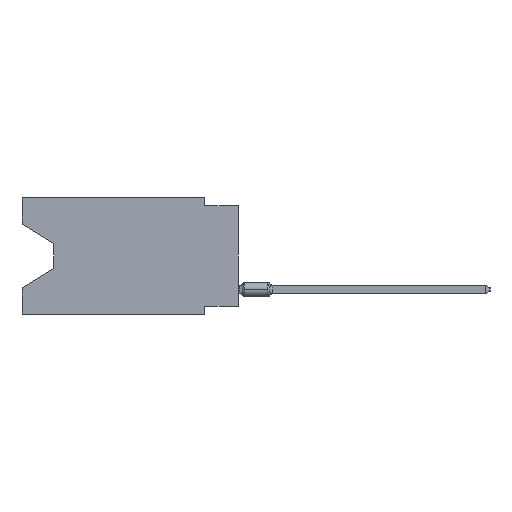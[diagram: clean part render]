
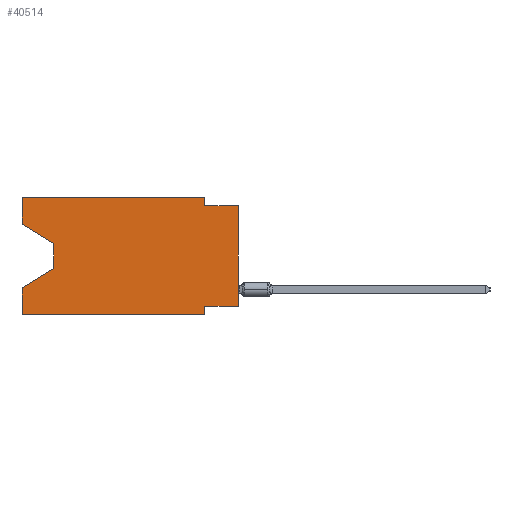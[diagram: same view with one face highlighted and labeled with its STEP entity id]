
A CAD part, left-side view. The second image highlights one B-rep face of the part: STEP entity #40514.
In plain terms, the highlighted planar face has unit normal (-1, 0, 0).
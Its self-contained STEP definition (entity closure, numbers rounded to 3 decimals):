
#3 = LINE ( 'NONE', #67822, #55058 ) ;
#1904 = DIRECTION ( 'NONE',  ( 0., -1., 0. ) ) ;
#2317 = ORIENTED_EDGE ( 'NONE', *, *, #14284, .F. ) ;
#2557 = VECTOR ( 'NONE', #18844, 1000. ) ;
#3692 = DIRECTION ( 'NONE',  ( 0., 0., -1. ) ) ;
#3915 = CARTESIAN_POINT ( 'NONE',  ( 0., 2.54, -8.255 ) ) ;
#7054 = CARTESIAN_POINT ( 'NONE',  ( 0., 0., -8.255 ) ) ;
#8529 = ORIENTED_EDGE ( 'NONE', *, *, #83714, .T. ) ;
#8626 = VECTOR ( 'NONE', #66168, 1000. ) ;
#8939 = DIRECTION ( 'NONE',  ( 0., 1., 0. ) ) ;
#9655 = VERTEX_POINT ( 'NONE', #47200 ) ;
#10917 = CARTESIAN_POINT ( 'NONE',  ( 0., 16.383, -2.038 ) ) ;
#12584 = CARTESIAN_POINT ( 'NONE',  ( 0., 16.383, 0. ) ) ;
#12741 = CARTESIAN_POINT ( 'NONE',  ( 0., 0., 0. ) ) ;
#12987 = ORIENTED_EDGE ( 'NONE', *, *, #36644, .F. ) ;
#13260 = LINE ( 'NONE', #43093, #8626 ) ;
#14284 = EDGE_CURVE ( 'NONE', #58173, #48306, #53150, .T. ) ;
#14728 = VERTEX_POINT ( 'NONE', #73076 ) ;
#16067 = VERTEX_POINT ( 'NONE', #92377 ) ;
#16090 = DIRECTION ( 'NONE',  ( 0., 0., 1. ) ) ;
#16483 = CARTESIAN_POINT ( 'NONE',  ( 0., 2.54, -0.635 ) ) ;
#18844 = DIRECTION ( 'NONE',  ( 0., -1., 0. ) ) ;
#21072 = EDGE_CURVE ( 'NONE', #58173, #93539, #63759, .T. ) ;
#21822 = EDGE_CURVE ( 'NONE', #61345, #56856, #24118, .T. ) ;
#22020 = VECTOR ( 'NONE', #79196, 1000. ) ;
#23165 = DIRECTION ( 'NONE',  ( 0., 0., -1. ) ) ;
#23327 = LINE ( 'NONE', #52690, #42760 ) ;
#24118 = LINE ( 'NONE', #75581, #46998 ) ;
#24303 = AXIS2_PLACEMENT_3D ( 'NONE', #12584, #35670, #84780 ) ;
#25368 = ORIENTED_EDGE ( 'NONE', *, *, #47477, .T. ) ;
#26266 = CARTESIAN_POINT ( 'NONE',  ( 0., 16.383, -2.038 ) ) ;
#27752 = VECTOR ( 'NONE', #3692, 1000. ) ;
#28472 = PLANE ( 'NONE',  #24303 ) ;
#29903 = VERTEX_POINT ( 'NONE', #81367 ) ;
#30614 = LINE ( 'NONE', #7054, #80110 ) ;
#32023 = EDGE_LOOP ( 'NONE', ( #59045, #74814, #25368, #32818, #40856, #78552, #12987, #8529, #39063, #64906, #34029, #2317 ) ) ;
#32818 = ORIENTED_EDGE ( 'NONE', *, *, #54060, .F. ) ;
#33780 = LINE ( 'NONE', #90544, #2557 ) ;
#34029 = ORIENTED_EDGE ( 'NONE', *, *, #73701, .F. ) ;
#35670 = DIRECTION ( 'NONE',  ( 1., 0., 0. ) ) ;
#36644 = EDGE_CURVE ( 'NONE', #80995, #50846, #30614, .T. ) ;
#38230 = DIRECTION ( 'NONE',  ( 0., 0., 1. ) ) ;
#39063 = ORIENTED_EDGE ( 'NONE', *, *, #92394, .F. ) ;
#40069 = VECTOR ( 'NONE', #38230, 1000. ) ;
#40514 = ADVANCED_FACE ( 'NONE', ( #94337 ), #28472, .F. ) ;
#40856 = ORIENTED_EDGE ( 'NONE', *, *, #75283, .T. ) ;
#42760 = VECTOR ( 'NONE', #16090, 1000. ) ;
#42927 = EDGE_CURVE ( 'NONE', #50846, #9655, #75851, .T. ) ;
#43093 = CARTESIAN_POINT ( 'NONE',  ( 0., 0., -0.635 ) ) ;
#45453 = CARTESIAN_POINT ( 'NONE',  ( 0., 16.383, 0. ) ) ;
#46998 = VECTOR ( 'NONE', #23165, 1000. ) ;
#47200 = CARTESIAN_POINT ( 'NONE',  ( 0., 2.54, -8.89 ) ) ;
#47477 = EDGE_CURVE ( 'NONE', #60207, #16067, #50353, .T. ) ;
#47492 = CARTESIAN_POINT ( 'NONE',  ( 0., 13.97, -3.505 ) ) ;
#48253 = VECTOR ( 'NONE', #84282, 1000. ) ;
#48306 = VERTEX_POINT ( 'NONE', #57218 ) ;
#50353 = LINE ( 'NONE', #56629, #22020 ) ;
#50846 = VERTEX_POINT ( 'NONE', #3915 ) ;
#52690 = CARTESIAN_POINT ( 'NONE',  ( 0., 16.383, 0. ) ) ;
#53150 = LINE ( 'NONE', #45453, #40069 ) ;
#54060 = EDGE_CURVE ( 'NONE', #14728, #16067, #23327, .T. ) ;
#54963 = LINE ( 'NONE', #76581, #48253 ) ;
#55058 = VECTOR ( 'NONE', #1904, 1000. ) ;
#56561 = DIRECTION ( 'NONE',  ( 0., -0.855, -0.519 ) ) ;
#56629 = CARTESIAN_POINT ( 'NONE',  ( 0., 13.97, -5.385 ) ) ;
#56856 = VERTEX_POINT ( 'NONE', #16483 ) ;
#57218 = CARTESIAN_POINT ( 'NONE',  ( 0., 16.383, 0. ) ) ;
#58173 = VERTEX_POINT ( 'NONE', #10917 ) ;
#59045 = ORIENTED_EDGE ( 'NONE', *, *, #21072, .T. ) ;
#60207 = VERTEX_POINT ( 'NONE', #94634 ) ;
#61345 = VERTEX_POINT ( 'NONE', #94509 ) ;
#63679 = CARTESIAN_POINT ( 'NONE',  ( 0., 0., -8.255 ) ) ;
#63759 = LINE ( 'NONE', #26266, #63815 ) ;
#63815 = VECTOR ( 'NONE', #56561, 1000. ) ;
#64906 = ORIENTED_EDGE ( 'NONE', *, *, #21822, .F. ) ;
#66129 = LINE ( 'NONE', #12741, #79376 ) ;
#66168 = DIRECTION ( 'NONE',  ( 0., -1., 0. ) ) ;
#67822 = CARTESIAN_POINT ( 'NONE',  ( 0., 16.383, -8.89 ) ) ;
#73076 = CARTESIAN_POINT ( 'NONE',  ( 0., 16.383, -8.89 ) ) ;
#73701 = EDGE_CURVE ( 'NONE', #48306, #61345, #33780, .T. ) ;
#74814 = ORIENTED_EDGE ( 'NONE', *, *, #82475, .T. ) ;
#75283 = EDGE_CURVE ( 'NONE', #14728, #9655, #3, .T. ) ;
#75581 = CARTESIAN_POINT ( 'NONE',  ( 0., 2.54, 0. ) ) ;
#75851 = LINE ( 'NONE', #83088, #27752 ) ;
#76581 = CARTESIAN_POINT ( 'NONE',  ( 0., 13.97, -3.505 ) ) ;
#78552 = ORIENTED_EDGE ( 'NONE', *, *, #42927, .F. ) ;
#79196 = DIRECTION ( 'NONE',  ( 0., 0.855, -0.519 ) ) ;
#79376 = VECTOR ( 'NONE', #79606, 1000. ) ;
#79606 = DIRECTION ( 'NONE',  ( 0., 0., 1. ) ) ;
#80110 = VECTOR ( 'NONE', #8939, 1000. ) ;
#80995 = VERTEX_POINT ( 'NONE', #63679 ) ;
#81367 = CARTESIAN_POINT ( 'NONE',  ( 0., 0., -0.635 ) ) ;
#82475 = EDGE_CURVE ( 'NONE', #93539, #60207, #54963, .T. ) ;
#83088 = CARTESIAN_POINT ( 'NONE',  ( 0., 2.54, -8.89 ) ) ;
#83714 = EDGE_CURVE ( 'NONE', #80995, #29903, #66129, .T. ) ;
#84282 = DIRECTION ( 'NONE',  ( 0., 0., -1. ) ) ;
#84780 = DIRECTION ( 'NONE',  ( 0., 0., -1. ) ) ;
#90544 = CARTESIAN_POINT ( 'NONE',  ( 0., 16.383, 0. ) ) ;
#92377 = CARTESIAN_POINT ( 'NONE',  ( 0., 16.383, -6.852 ) ) ;
#92394 = EDGE_CURVE ( 'NONE', #56856, #29903, #13260, .T. ) ;
#93539 = VERTEX_POINT ( 'NONE', #47492 ) ;
#94337 = FACE_OUTER_BOUND ( 'NONE', #32023, .T. ) ;
#94509 = CARTESIAN_POINT ( 'NONE',  ( 0., 2.54, 0. ) ) ;
#94634 = CARTESIAN_POINT ( 'NONE',  ( 0., 13.97, -5.385 ) ) ;
